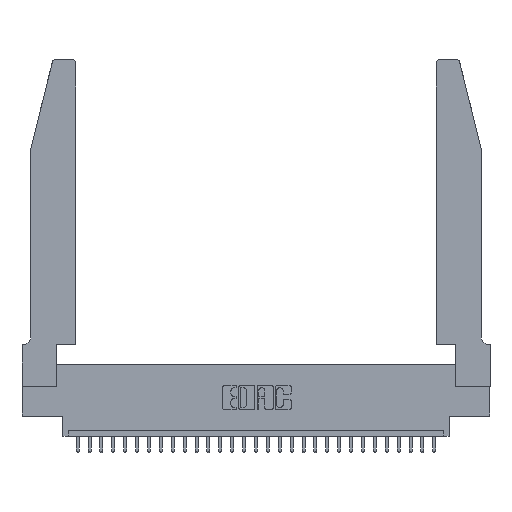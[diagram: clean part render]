
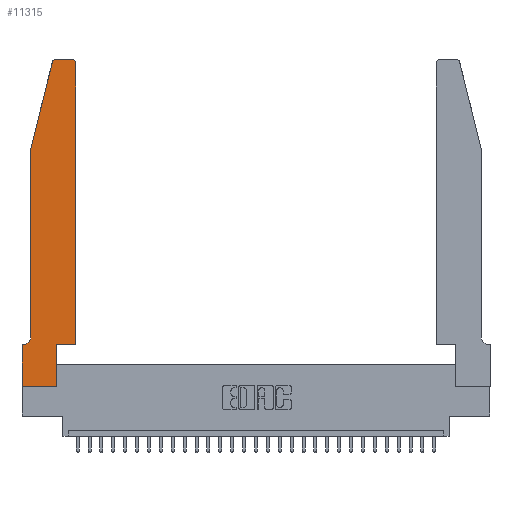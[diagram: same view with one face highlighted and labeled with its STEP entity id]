
A CAD part, top view. The second image highlights one B-rep face of the part: STEP entity #11315.
In plain terms, the highlighted planar face has unit normal (0, 0, 1).
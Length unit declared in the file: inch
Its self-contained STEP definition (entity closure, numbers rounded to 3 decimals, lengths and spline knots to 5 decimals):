
#333 = EDGE_CURVE ( 'NONE', #24256, #28522, #19865, .T. ) ;
#418 = CARTESIAN_POINT ( 'NONE',  ( 0.284, 2.75, 0.37 ) ) ;
#481 = CARTESIAN_POINT ( 'NONE',  ( 0., 0., 0.37 ) ) ;
#492 = CIRCLE ( 'NONE', #15163, 0.03 ) ;
#611 = CARTESIAN_POINT ( 'NONE',  ( 0.4505, 0.35, 0.37 ) ) ;
#876 = EDGE_CURVE ( 'NONE', #10646, #23120, #1559, .T. ) ;
#985 = LINE ( 'NONE', #12973, #6708 ) ;
#1122 = AXIS2_PLACEMENT_3D ( 'NONE', #2589, #25515, #18561 ) ;
#1225 = CARTESIAN_POINT ( 'NONE',  ( 0.284, 2.72, 0.37 ) ) ;
#1422 = LINE ( 'NONE', #23775, #15768 ) ;
#1559 = LINE ( 'NONE', #16943, #21261 ) ;
#2472 = PLANE ( 'NONE',  #1122 ) ;
#2589 = CARTESIAN_POINT ( 'NONE',  ( 0., 0.35, 0.37 ) ) ;
#2841 = CARTESIAN_POINT ( 'NONE',  ( 0.0755, 2., 0.37 ) ) ;
#3321 = DIRECTION ( 'NONE',  ( 0., 0., -1. ) ) ;
#3378 = CARTESIAN_POINT ( 'NONE',  ( 0.2865, 0.35, 0.37 ) ) ;
#3795 = DIRECTION ( 'NONE',  ( -0.239, -0.971, 0. ) ) ;
#4644 = ORIENTED_EDGE ( 'NONE', *, *, #333, .T. ) ;
#4913 = DIRECTION ( 'NONE',  ( 0., 1., 0. ) ) ;
#5019 = AXIS2_PLACEMENT_3D ( 'NONE', #5401, #3321, #14931 ) ;
#5401 = CARTESIAN_POINT ( 'NONE',  ( 0.0055, 0.42, 0.37 ) ) ;
#6049 = LINE ( 'NONE', #29297, #8182 ) ;
#6357 = CARTESIAN_POINT ( 'NONE',  ( 0.0755, 2., 0.37 ) ) ;
#6708 = VECTOR ( 'NONE', #12876, 39.37008 ) ;
#6760 = EDGE_CURVE ( 'NONE', #20240, #15660, #11084, .T. ) ;
#6934 = CARTESIAN_POINT ( 'NONE',  ( 0.4505, 0.35, 0.37 ) ) ;
#7512 = ORIENTED_EDGE ( 'NONE', *, *, #23071, .T. ) ;
#7553 = ORIENTED_EDGE ( 'NONE', *, *, #21079, .T. ) ;
#8059 = VERTEX_POINT ( 'NONE', #25453 ) ;
#8182 = VECTOR ( 'NONE', #8307, 39.37008 ) ;
#8307 = DIRECTION ( 'NONE',  ( -1., 0., 0. ) ) ;
#9094 = EDGE_LOOP ( 'NONE', ( #18660, #21625, #24933, #7512, #4644, #18868, #28491, #18300, #7553, #24396, #26380, #13987 ) ) ;
#9279 = DIRECTION ( 'NONE',  ( 1., 0., 0. ) ) ;
#10129 = DIRECTION ( 'NONE',  ( 0., 1., 0. ) ) ;
#10182 = EDGE_CURVE ( 'NONE', #28522, #25971, #1422, .T. ) ;
#10646 = VERTEX_POINT ( 'NONE', #3378 ) ;
#11084 = LINE ( 'NONE', #29660, #28702 ) ;
#11182 = EDGE_CURVE ( 'NONE', #24368, #19510, #20760, .T. ) ;
#11315 = ADVANCED_FACE ( 'NONE', ( #23990 ), #2472, .T. ) ;
#11504 = CARTESIAN_POINT ( 'NONE',  ( 0.4205, 2.72, 0.37 ) ) ;
#11889 = LINE ( 'NONE', #6934, #22650 ) ;
#11926 = EDGE_CURVE ( 'NONE', #25971, #20240, #985, .T. ) ;
#12292 = VERTEX_POINT ( 'NONE', #418 ) ;
#12430 = DIRECTION ( 'NONE',  ( 0., 0., 1. ) ) ;
#12876 = DIRECTION ( 'NONE',  ( 0., -1., 0. ) ) ;
#12973 = CARTESIAN_POINT ( 'NONE',  ( 0., 0., 0.37 ) ) ;
#13115 = CARTESIAN_POINT ( 'NONE',  ( 0.25487, 2.72718, 0.37 ) ) ;
#13152 = VECTOR ( 'NONE', #10129, 39.37008 ) ;
#13351 = CARTESIAN_POINT ( 'NONE',  ( 0.4505, 2.72, 0.37 ) ) ;
#13393 = CARTESIAN_POINT ( 'NONE',  ( 0.0755, 2., 0.37 ) ) ;
#13916 = EDGE_CURVE ( 'NONE', #21233, #8059, #492, .T. ) ;
#13987 = ORIENTED_EDGE ( 'NONE', *, *, #13916, .T. ) ;
#14661 = VECTOR ( 'NONE', #3795, 39.37008 ) ;
#14725 = DIRECTION ( 'NONE',  ( 1., 0., 0. ) ) ;
#14726 = CARTESIAN_POINT ( 'NONE',  ( 0.0755, 0.42, 0.37 ) ) ;
#14931 = DIRECTION ( 'NONE',  ( -1., 0., 0. ) ) ;
#15158 = CARTESIAN_POINT ( 'NONE',  ( 0.2865, 0.35, 0.37 ) ) ;
#15163 = AXIS2_PLACEMENT_3D ( 'NONE', #11504, #27580, #9279 ) ;
#15446 = AXIS2_PLACEMENT_3D ( 'NONE', #1225, #12430, #28796 ) ;
#15660 = VERTEX_POINT ( 'NONE', #19556 ) ;
#15768 = VECTOR ( 'NONE', #28324, 39.37008 ) ;
#16655 = DIRECTION ( 'NONE',  ( 0., -1., 0. ) ) ;
#16733 = VECTOR ( 'NONE', #16655, 39.37008 ) ;
#16943 = CARTESIAN_POINT ( 'NONE',  ( 0.4505, 0.35, 0.37 ) ) ;
#17243 = CIRCLE ( 'NONE', #15446, 0.03 ) ;
#17688 = EDGE_CURVE ( 'NONE', #23120, #21233, #11889, .T. ) ;
#17691 = DIRECTION ( 'NONE',  ( 1., 0., 0. ) ) ;
#18300 = ORIENTED_EDGE ( 'NONE', *, *, #6760, .T. ) ;
#18339 = CARTESIAN_POINT ( 'NONE',  ( 0.0055, 0.35, 0.37 ) ) ;
#18561 = DIRECTION ( 'NONE',  ( 1., 0., 0. ) ) ;
#18660 = ORIENTED_EDGE ( 'NONE', *, *, #19999, .T. ) ;
#18868 = ORIENTED_EDGE ( 'NONE', *, *, #10182, .T. ) ;
#19132 = CARTESIAN_POINT ( 'NONE',  ( 0., 0.35, 0.37 ) ) ;
#19510 = VERTEX_POINT ( 'NONE', #6357 ) ;
#19556 = CARTESIAN_POINT ( 'NONE',  ( 0.2865, 0., 0.37 ) ) ;
#19865 = CIRCLE ( 'NONE', #5019, 0.07 ) ;
#19999 = EDGE_CURVE ( 'NONE', #8059, #12292, #6049, .T. ) ;
#20240 = VERTEX_POINT ( 'NONE', #481 ) ;
#20760 = LINE ( 'NONE', #13393, #14661 ) ;
#21079 = EDGE_CURVE ( 'NONE', #15660, #10646, #28929, .T. ) ;
#21233 = VERTEX_POINT ( 'NONE', #13351 ) ;
#21261 = VECTOR ( 'NONE', #14725, 39.37008 ) ;
#21625 = ORIENTED_EDGE ( 'NONE', *, *, #28714, .T. ) ;
#22650 = VECTOR ( 'NONE', #4913, 39.37008 ) ;
#23071 = EDGE_CURVE ( 'NONE', #19510, #24256, #25712, .T. ) ;
#23120 = VERTEX_POINT ( 'NONE', #611 ) ;
#23775 = CARTESIAN_POINT ( 'NONE',  ( 0.0755, 0.35, 0.37 ) ) ;
#23990 = FACE_OUTER_BOUND ( 'NONE', #9094, .T. ) ;
#24256 = VERTEX_POINT ( 'NONE', #14726 ) ;
#24368 = VERTEX_POINT ( 'NONE', #13115 ) ;
#24396 = ORIENTED_EDGE ( 'NONE', *, *, #876, .T. ) ;
#24933 = ORIENTED_EDGE ( 'NONE', *, *, #11182, .T. ) ;
#25453 = CARTESIAN_POINT ( 'NONE',  ( 0.4205, 2.75, 0.37 ) ) ;
#25515 = DIRECTION ( 'NONE',  ( 0., 0., 1. ) ) ;
#25712 = LINE ( 'NONE', #2841, #16733 ) ;
#25971 = VERTEX_POINT ( 'NONE', #19132 ) ;
#26380 = ORIENTED_EDGE ( 'NONE', *, *, #17688, .T. ) ;
#27580 = DIRECTION ( 'NONE',  ( 0., 0., 1. ) ) ;
#28324 = DIRECTION ( 'NONE',  ( -1., 0., 0. ) ) ;
#28491 = ORIENTED_EDGE ( 'NONE', *, *, #11926, .T. ) ;
#28522 = VERTEX_POINT ( 'NONE', #18339 ) ;
#28702 = VECTOR ( 'NONE', #17691, 39.37008 ) ;
#28714 = EDGE_CURVE ( 'NONE', #12292, #24368, #17243, .T. ) ;
#28796 = DIRECTION ( 'NONE',  ( 1., 0., 0. ) ) ;
#28929 = LINE ( 'NONE', #15158, #13152 ) ;
#29297 = CARTESIAN_POINT ( 'NONE',  ( 0.2605, 2.75, 0.37 ) ) ;
#29660 = CARTESIAN_POINT ( 'NONE',  ( 0., 0., 0.37 ) ) ;
